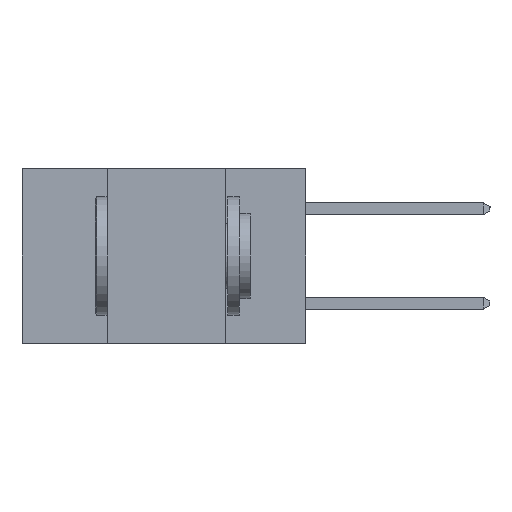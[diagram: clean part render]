
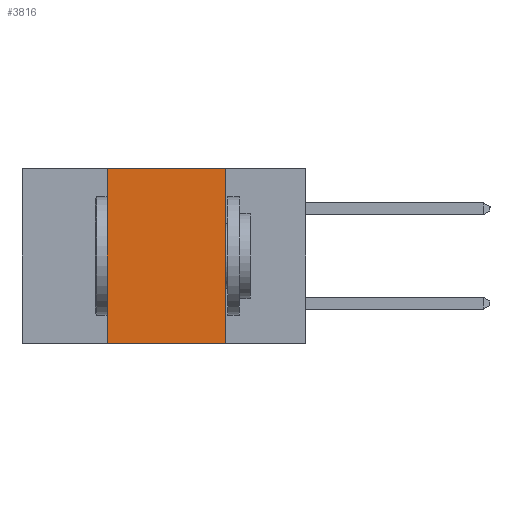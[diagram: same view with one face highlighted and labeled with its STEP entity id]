
A CAD part, left-side view. The second image highlights one B-rep face of the part: STEP entity #3816.
In plain terms, the highlighted planar face has unit normal (-1, 0, 0).
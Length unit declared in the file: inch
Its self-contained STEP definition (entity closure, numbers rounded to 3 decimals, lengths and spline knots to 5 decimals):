
#14 = LINE ( 'NONE', #2744, #14358 ) ;
#718 = LINE ( 'NONE', #11025, #5170 ) ;
#802 = DIRECTION ( 'NONE',  ( 0., -1., 0. ) ) ;
#1276 = CARTESIAN_POINT ( 'NONE',  ( 0., 0.42, 0. ) ) ;
#1707 = FACE_OUTER_BOUND ( 'NONE', #10955, .T. ) ;
#1876 = EDGE_CURVE ( 'NONE', #15140, #8828, #718, .T. ) ;
#2744 = CARTESIAN_POINT ( 'NONE',  ( 0., 0.17, -0.37 ) ) ;
#3273 = EDGE_CURVE ( 'NONE', #5651, #8828, #14, .T. ) ;
#3686 = LINE ( 'NONE', #13944, #6331 ) ;
#3816 = ADVANCED_FACE ( 'NONE', ( #1707 ), #15721, .F. ) ;
#4679 = CARTESIAN_POINT ( 'NONE',  ( 0., 0.17, -0.37 ) ) ;
#5170 = VECTOR ( 'NONE', #802, 39.37008 ) ;
#5397 = ORIENTED_EDGE ( 'NONE', *, *, #1876, .T. ) ;
#5651 = VERTEX_POINT ( 'NONE', #11181 ) ;
#5814 = CARTESIAN_POINT ( 'NONE',  ( 0., 0.6, 0. ) ) ;
#5836 = VERTEX_POINT ( 'NONE', #1276 ) ;
#6331 = VECTOR ( 'NONE', #16310, 39.37008 ) ;
#6816 = CARTESIAN_POINT ( 'NONE',  ( 0., 0.6, 0. ) ) ;
#7220 = EDGE_CURVE ( 'NONE', #15140, #5836, #3686, .T. ) ;
#7269 = CARTESIAN_POINT ( 'NONE',  ( 0., 0.42, -0.37 ) ) ;
#7621 = ORIENTED_EDGE ( 'NONE', *, *, #3273, .F. ) ;
#7770 = AXIS2_PLACEMENT_3D ( 'NONE', #6816, #9680, #11954 ) ;
#8121 = ORIENTED_EDGE ( 'NONE', *, *, #15433, .F. ) ;
#8828 = VERTEX_POINT ( 'NONE', #4679 ) ;
#9314 = ORIENTED_EDGE ( 'NONE', *, *, #7220, .F. ) ;
#9680 = DIRECTION ( 'NONE',  ( 1., 0., 0. ) ) ;
#9954 = DIRECTION ( 'NONE',  ( 0., -1., 0. ) ) ;
#10034 = LINE ( 'NONE', #5814, #16411 ) ;
#10955 = EDGE_LOOP ( 'NONE', ( #7621, #8121, #9314, #5397 ) ) ;
#11025 = CARTESIAN_POINT ( 'NONE',  ( 0., 0.6, -0.37 ) ) ;
#11181 = CARTESIAN_POINT ( 'NONE',  ( 0., 0.17, 0. ) ) ;
#11954 = DIRECTION ( 'NONE',  ( 0., 0., -1. ) ) ;
#13944 = CARTESIAN_POINT ( 'NONE',  ( 0., 0.42, -0.37 ) ) ;
#14358 = VECTOR ( 'NONE', #15335, 39.37008 ) ;
#15140 = VERTEX_POINT ( 'NONE', #7269 ) ;
#15335 = DIRECTION ( 'NONE',  ( 0., 0., -1. ) ) ;
#15433 = EDGE_CURVE ( 'NONE', #5836, #5651, #10034, .T. ) ;
#15721 = PLANE ( 'NONE',  #7770 ) ;
#16310 = DIRECTION ( 'NONE',  ( 0., 0., 1. ) ) ;
#16411 = VECTOR ( 'NONE', #9954, 39.37008 ) ;
